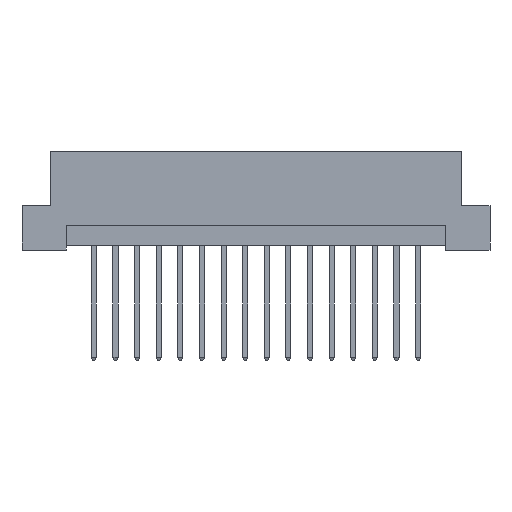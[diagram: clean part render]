
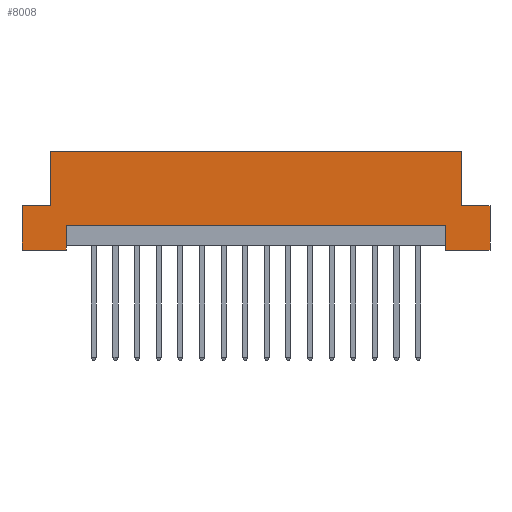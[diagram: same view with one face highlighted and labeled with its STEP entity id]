
A CAD part, front view. The second image highlights one B-rep face of the part: STEP entity #8008.
In plain terms, the highlighted planar face has unit normal (0, -1, 0).
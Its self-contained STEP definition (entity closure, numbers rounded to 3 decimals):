
#12 = DIRECTION ( 'NONE',  ( 1., 0., 0. ) ) ;
#48 = ORIENTED_EDGE ( 'NONE', *, *, #4325, .T. ) ;
#131 = DIRECTION ( 'NONE',  ( 1., 0., 0. ) ) ;
#236 = CARTESIAN_POINT ( 'NONE',  ( 22.3, 0., 2.9 ) ) ;
#288 = VERTEX_POINT ( 'NONE', #9843 ) ;
#306 = DIRECTION ( 'NONE',  ( 0., 0., 1. ) ) ;
#554 = DIRECTION ( 'NONE',  ( 1., 0., 0. ) ) ;
#569 = VECTOR ( 'NONE', #2323, 1000. ) ;
#598 = VECTOR ( 'NONE', #131, 1000. ) ;
#703 = CARTESIAN_POINT ( 'NONE',  ( 27.5, 0., 5.2 ) ) ;
#1086 = EDGE_CURVE ( 'NONE', #3714, #288, #8587, .T. ) ;
#1187 = CARTESIAN_POINT ( 'NONE',  ( 24.2, 0., 11.6 ) ) ;
#1382 = ORIENTED_EDGE ( 'NONE', *, *, #5101, .F. ) ;
#1399 = VERTEX_POINT ( 'NONE', #6575 ) ;
#1488 = ORIENTED_EDGE ( 'NONE', *, *, #4147, .F. ) ;
#1499 = VERTEX_POINT ( 'NONE', #6903 ) ;
#1586 = FACE_OUTER_BOUND ( 'NONE', #3153, .T. ) ;
#1607 = LINE ( 'NONE', #8886, #3723 ) ;
#1686 = CARTESIAN_POINT ( 'NONE',  ( -27.5, 0., 11.6 ) ) ;
#1817 = ORIENTED_EDGE ( 'NONE', *, *, #7873, .F. ) ;
#2164 = CARTESIAN_POINT ( 'NONE',  ( 24.2, 0., 5.2 ) ) ;
#2204 = VERTEX_POINT ( 'NONE', #1187 ) ;
#2271 = DIRECTION ( 'NONE',  ( 0., 0., 1. ) ) ;
#2323 = DIRECTION ( 'NONE',  ( -1., 0., 0. ) ) ;
#2370 = VECTOR ( 'NONE', #8843, 1000. ) ;
#2410 = VECTOR ( 'NONE', #6167, 1000. ) ;
#2463 = ORIENTED_EDGE ( 'NONE', *, *, #6096, .F. ) ;
#2547 = VECTOR ( 'NONE', #6651, 1000. ) ;
#2711 = VECTOR ( 'NONE', #6597, 1000. ) ;
#2936 = VECTOR ( 'NONE', #7881, 1000. ) ;
#2952 = CARTESIAN_POINT ( 'NONE',  ( 27.5, 0., 0. ) ) ;
#3153 = EDGE_LOOP ( 'NONE', ( #1382, #48, #7423, #7387, #1488, #6515, #3405, #2463, #4643, #5255, #1817, #4522 ) ) ;
#3405 = ORIENTED_EDGE ( 'NONE', *, *, #4186, .F. ) ;
#3642 = CARTESIAN_POINT ( 'NONE',  ( 27.5, 0., 0. ) ) ;
#3650 = EDGE_CURVE ( 'NONE', #4829, #3714, #8821, .T. ) ;
#3714 = VERTEX_POINT ( 'NONE', #9551 ) ;
#3723 = VECTOR ( 'NONE', #7883, 1000. ) ;
#3735 = LINE ( 'NONE', #7025, #569 ) ;
#4063 = LINE ( 'NONE', #7457, #2711 ) ;
#4128 = VECTOR ( 'NONE', #554, 1000. ) ;
#4147 = EDGE_CURVE ( 'NONE', #10146, #6463, #9525, .T. ) ;
#4186 = EDGE_CURVE ( 'NONE', #8798, #2204, #9687, .T. ) ;
#4325 = EDGE_CURVE ( 'NONE', #8063, #1399, #6580, .T. ) ;
#4353 = CARTESIAN_POINT ( 'NONE',  ( -27.5, 0., 0. ) ) ;
#4522 = ORIENTED_EDGE ( 'NONE', *, *, #6122, .F. ) ;
#4569 = AXIS2_PLACEMENT_3D ( 'NONE', #6175, #5428, #2271 ) ;
#4643 = ORIENTED_EDGE ( 'NONE', *, *, #1086, .F. ) ;
#4829 = VERTEX_POINT ( 'NONE', #4353 ) ;
#5057 = CARTESIAN_POINT ( 'NONE',  ( 22.3, 0., 0.5 ) ) ;
#5101 = EDGE_CURVE ( 'NONE', #8063, #1499, #1607, .T. ) ;
#5255 = ORIENTED_EDGE ( 'NONE', *, *, #3650, .F. ) ;
#5428 = DIRECTION ( 'NONE',  ( 0., 1., 0. ) ) ;
#5659 = CARTESIAN_POINT ( 'NONE',  ( -24.2, 0., 5.2 ) ) ;
#5782 = VERTEX_POINT ( 'NONE', #6890 ) ;
#5814 = VECTOR ( 'NONE', #12, 1000. ) ;
#5914 = VECTOR ( 'NONE', #306, 1000. ) ;
#5989 = CARTESIAN_POINT ( 'NONE',  ( -24.2, 0., 11.6 ) ) ;
#6096 = EDGE_CURVE ( 'NONE', #288, #8798, #8924, .T. ) ;
#6122 = EDGE_CURVE ( 'NONE', #1499, #5782, #4063, .T. ) ;
#6161 = LINE ( 'NONE', #8538, #2370 ) ;
#6167 = DIRECTION ( 'NONE',  ( 0., 0., -1. ) ) ;
#6175 = CARTESIAN_POINT ( 'NONE',  ( -27.5, 0., 11.6 ) ) ;
#6248 = EDGE_CURVE ( 'NONE', #10146, #2204, #7513, .T. ) ;
#6359 = EDGE_CURVE ( 'NONE', #7728, #1399, #6161, .T. ) ;
#6463 = VERTEX_POINT ( 'NONE', #703 ) ;
#6515 = ORIENTED_EDGE ( 'NONE', *, *, #6248, .T. ) ;
#6575 = CARTESIAN_POINT ( 'NONE',  ( 22.3, 0., 0. ) ) ;
#6580 = LINE ( 'NONE', #5057, #6905 ) ;
#6597 = DIRECTION ( 'NONE',  ( 0., 0., -1. ) ) ;
#6651 = DIRECTION ( 'NONE',  ( 0., 0., 1. ) ) ;
#6890 = CARTESIAN_POINT ( 'NONE',  ( -22.3, 0., 0. ) ) ;
#6903 = CARTESIAN_POINT ( 'NONE',  ( -22.3, 0., 2.9 ) ) ;
#6905 = VECTOR ( 'NONE', #9837, 1000. ) ;
#6917 = CARTESIAN_POINT ( 'NONE',  ( -27.5, 0., 5.2 ) ) ;
#7025 = CARTESIAN_POINT ( 'NONE',  ( -27.5, 0., 0. ) ) ;
#7387 = ORIENTED_EDGE ( 'NONE', *, *, #9742, .F. ) ;
#7423 = ORIENTED_EDGE ( 'NONE', *, *, #6359, .F. ) ;
#7457 = CARTESIAN_POINT ( 'NONE',  ( -22.3, 0., 0.5 ) ) ;
#7513 = LINE ( 'NONE', #2164, #5914 ) ;
#7728 = VERTEX_POINT ( 'NONE', #3642 ) ;
#7873 = EDGE_CURVE ( 'NONE', #5782, #4829, #3735, .T. ) ;
#7881 = DIRECTION ( 'NONE',  ( 0., 0., 1. ) ) ;
#7883 = DIRECTION ( 'NONE',  ( -1., 0., 0. ) ) ;
#8008 = ADVANCED_FACE ( 'NONE', ( #1586 ), #10159, .F. ) ;
#8063 = VERTEX_POINT ( 'NONE', #236 ) ;
#8538 = CARTESIAN_POINT ( 'NONE',  ( -27.5, 0., 0. ) ) ;
#8587 = LINE ( 'NONE', #6917, #4128 ) ;
#8717 = CARTESIAN_POINT ( 'NONE',  ( -27.5, 0., 0. ) ) ;
#8741 = CARTESIAN_POINT ( 'NONE',  ( 27.5, 0., 5.2 ) ) ;
#8798 = VERTEX_POINT ( 'NONE', #5989 ) ;
#8821 = LINE ( 'NONE', #8717, #2936 ) ;
#8843 = DIRECTION ( 'NONE',  ( -1., 0., 0. ) ) ;
#8886 = CARTESIAN_POINT ( 'NONE',  ( 22.3, 0., 2.9 ) ) ;
#8924 = LINE ( 'NONE', #5659, #2547 ) ;
#9525 = LINE ( 'NONE', #8741, #5814 ) ;
#9551 = CARTESIAN_POINT ( 'NONE',  ( -27.5, 0., 5.2 ) ) ;
#9687 = LINE ( 'NONE', #1686, #598 ) ;
#9742 = EDGE_CURVE ( 'NONE', #6463, #7728, #10298, .T. ) ;
#9837 = DIRECTION ( 'NONE',  ( 0., 0., -1. ) ) ;
#9843 = CARTESIAN_POINT ( 'NONE',  ( -24.2, 0., 5.2 ) ) ;
#9873 = CARTESIAN_POINT ( 'NONE',  ( 24.2, 0., 5.2 ) ) ;
#10146 = VERTEX_POINT ( 'NONE', #9873 ) ;
#10159 = PLANE ( 'NONE',  #4569 ) ;
#10298 = LINE ( 'NONE', #2952, #2410 ) ;
